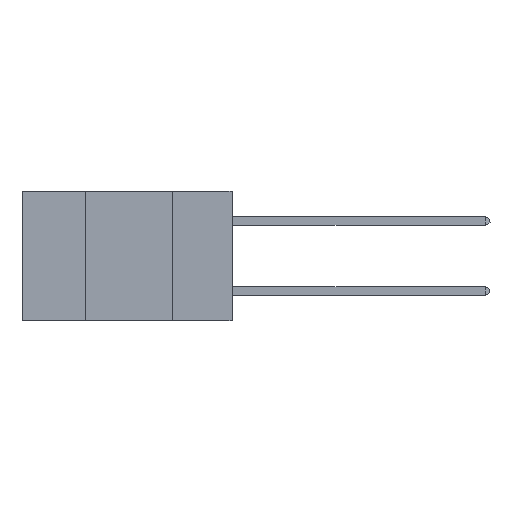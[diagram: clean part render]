
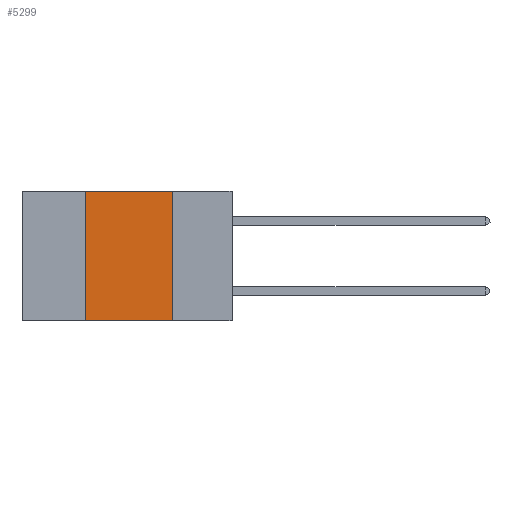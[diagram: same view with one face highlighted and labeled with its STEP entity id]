
A CAD part, left-side view. The second image highlights one B-rep face of the part: STEP entity #5299.
In plain terms, the highlighted planar face has unit normal (-1, 0, 0).
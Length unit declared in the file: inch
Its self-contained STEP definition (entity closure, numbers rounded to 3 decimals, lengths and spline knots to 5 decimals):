
#724 = PLANE ( 'NONE',  #1506 ) ;
#1123 = CARTESIAN_POINT ( 'NONE',  ( 0., 0.42, -0.37 ) ) ;
#1506 = AXIS2_PLACEMENT_3D ( 'NONE', #3762, #13356, #2109 ) ;
#2082 = ORIENTED_EDGE ( 'NONE', *, *, #6460, .T. ) ;
#2109 = DIRECTION ( 'NONE',  ( 0., 0., -1. ) ) ;
#2178 = CARTESIAN_POINT ( 'NONE',  ( 0., 0.6, -0.37 ) ) ;
#2199 = ORIENTED_EDGE ( 'NONE', *, *, #7869, .F. ) ;
#2825 = VERTEX_POINT ( 'NONE', #1123 ) ;
#3179 = VECTOR ( 'NONE', #14717, 39.37008 ) ;
#3762 = CARTESIAN_POINT ( 'NONE',  ( 0., 0.6, 0. ) ) ;
#4063 = CARTESIAN_POINT ( 'NONE',  ( 0., 0.6, 0. ) ) ;
#4613 = CARTESIAN_POINT ( 'NONE',  ( 0., 0.17, -0.37 ) ) ;
#5216 = CARTESIAN_POINT ( 'NONE',  ( 0., 0.17, 0. ) ) ;
#5299 = ADVANCED_FACE ( 'NONE', ( #15515 ), #724, .F. ) ;
#5515 = LINE ( 'NONE', #11414, #10033 ) ;
#6460 = EDGE_CURVE ( 'NONE', #2825, #7573, #11777, .T. ) ;
#7376 = ORIENTED_EDGE ( 'NONE', *, *, #10485, .F. ) ;
#7573 = VERTEX_POINT ( 'NONE', #4613 ) ;
#7869 = EDGE_CURVE ( 'NONE', #10286, #13074, #13608, .T. ) ;
#7993 = DIRECTION ( 'NONE',  ( 0., -1., 0. ) ) ;
#8047 = CARTESIAN_POINT ( 'NONE',  ( 0., 0.17, 0. ) ) ;
#9406 = VECTOR ( 'NONE', #7993, 39.37008 ) ;
#10033 = VECTOR ( 'NONE', #12630, 39.37008 ) ;
#10286 = VERTEX_POINT ( 'NONE', #14681 ) ;
#10485 = EDGE_CURVE ( 'NONE', #13074, #7573, #12822, .T. ) ;
#11278 = EDGE_CURVE ( 'NONE', #2825, #10286, #5515, .T. ) ;
#11414 = CARTESIAN_POINT ( 'NONE',  ( 0., 0.42, 0. ) ) ;
#11777 = LINE ( 'NONE', #2178, #9406 ) ;
#12630 = DIRECTION ( 'NONE',  ( 0., 0., 1. ) ) ;
#12822 = LINE ( 'NONE', #5216, #3179 ) ;
#13074 = VERTEX_POINT ( 'NONE', #8047 ) ;
#13356 = DIRECTION ( 'NONE',  ( 1., 0., 0. ) ) ;
#13434 = ORIENTED_EDGE ( 'NONE', *, *, #11278, .F. ) ;
#13608 = LINE ( 'NONE', #4063, #14468 ) ;
#13609 = DIRECTION ( 'NONE',  ( 0., -1., 0. ) ) ;
#14468 = VECTOR ( 'NONE', #13609, 39.37008 ) ;
#14681 = CARTESIAN_POINT ( 'NONE',  ( 0., 0.42, 0. ) ) ;
#14717 = DIRECTION ( 'NONE',  ( 0., 0., -1. ) ) ;
#15515 = FACE_OUTER_BOUND ( 'NONE', #16304, .T. ) ;
#16304 = EDGE_LOOP ( 'NONE', ( #7376, #2199, #13434, #2082 ) ) ;
